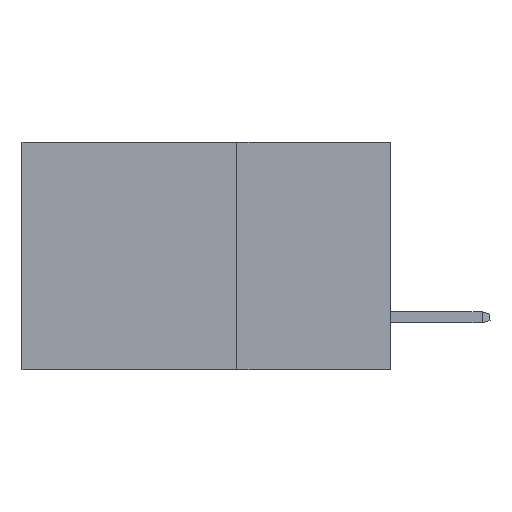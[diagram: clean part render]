
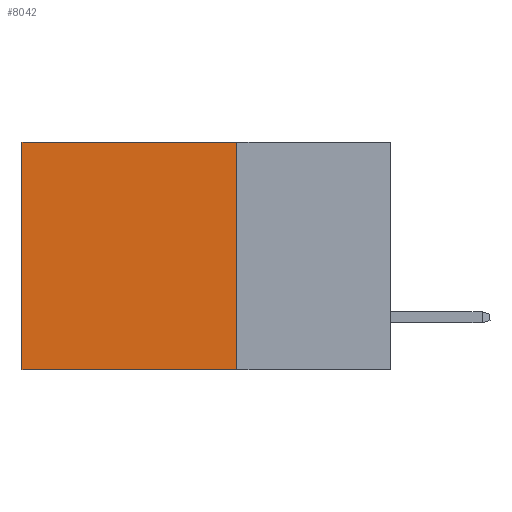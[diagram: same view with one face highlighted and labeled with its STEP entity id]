
A CAD part, left-side view. The second image highlights one B-rep face of the part: STEP entity #8042.
In plain terms, the highlighted planar face has unit normal (-1, 0, 0).
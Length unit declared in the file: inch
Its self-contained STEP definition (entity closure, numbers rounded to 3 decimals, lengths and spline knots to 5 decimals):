
#10 = LINE ( 'NONE', #5306, #6975 ) ;
#250 = CARTESIAN_POINT ( 'NONE',  ( 0.2875, 0.6, 0. ) ) ;
#1092 = VECTOR ( 'NONE', #1236, 39.37008 ) ;
#1236 = DIRECTION ( 'NONE',  ( 0., 0., -1. ) ) ;
#1239 = CARTESIAN_POINT ( 'NONE',  ( 0.2875, 0.6, -0.37 ) ) ;
#2367 = VECTOR ( 'NONE', #9723, 39.37008 ) ;
#2825 = ORIENTED_EDGE ( 'NONE', *, *, #8711, .T. ) ;
#2900 = ORIENTED_EDGE ( 'NONE', *, *, #8408, .F. ) ;
#3017 = ORIENTED_EDGE ( 'NONE', *, *, #7733, .F. ) ;
#3264 = VERTEX_POINT ( 'NONE', #4127 ) ;
#3443 = ORIENTED_EDGE ( 'NONE', *, *, #3919, .T. ) ;
#3919 = EDGE_CURVE ( 'NONE', #11159, #7551, #10567, .T. ) ;
#3991 = PLANE ( 'NONE',  #8939 ) ;
#4127 = CARTESIAN_POINT ( 'NONE',  ( 0.2875, 0.25, -0.37 ) ) ;
#4461 = LINE ( 'NONE', #8911, #2367 ) ;
#4876 = DIRECTION ( 'NONE',  ( 1., 0., 0. ) ) ;
#5306 = CARTESIAN_POINT ( 'NONE',  ( 0.2875, 0.25, 0. ) ) ;
#5378 = EDGE_LOOP ( 'NONE', ( #2825, #2900, #3017, #3443 ) ) ;
#5619 = VERTEX_POINT ( 'NONE', #1239 ) ;
#6635 = CARTESIAN_POINT ( 'NONE',  ( 0.2875, 0.25, 0. ) ) ;
#6873 = CARTESIAN_POINT ( 'NONE',  ( 0.2875, 0.6, 0. ) ) ;
#6975 = VECTOR ( 'NONE', #11169, 39.37008 ) ;
#7551 = VERTEX_POINT ( 'NONE', #6873 ) ;
#7733 = EDGE_CURVE ( 'NONE', #11159, #3264, #10, .T. ) ;
#8042 = ADVANCED_FACE ( 'NONE', ( #8068 ), #3991, .F. ) ;
#8068 = FACE_OUTER_BOUND ( 'NONE', #5378, .T. ) ;
#8408 = EDGE_CURVE ( 'NONE', #3264, #5619, #4461, .T. ) ;
#8459 = LINE ( 'NONE', #250, #1092 ) ;
#8550 = CARTESIAN_POINT ( 'NONE',  ( 0.2875, 0.25, 0. ) ) ;
#8711 = EDGE_CURVE ( 'NONE', #7551, #5619, #8459, .T. ) ;
#8911 = CARTESIAN_POINT ( 'NONE',  ( 0.2875, 0.25, -0.37 ) ) ;
#8939 = AXIS2_PLACEMENT_3D ( 'NONE', #6635, #4876, #10791 ) ;
#9723 = DIRECTION ( 'NONE',  ( 0., 1., 0. ) ) ;
#10320 = VECTOR ( 'NONE', #10843, 39.37008 ) ;
#10567 = LINE ( 'NONE', #10810, #10320 ) ;
#10791 = DIRECTION ( 'NONE',  ( 0., 0., -1. ) ) ;
#10810 = CARTESIAN_POINT ( 'NONE',  ( 0.2875, 0.25, 0. ) ) ;
#10843 = DIRECTION ( 'NONE',  ( 0., 1., 0. ) ) ;
#11159 = VERTEX_POINT ( 'NONE', #8550 ) ;
#11169 = DIRECTION ( 'NONE',  ( 0., 0., -1. ) ) ;
